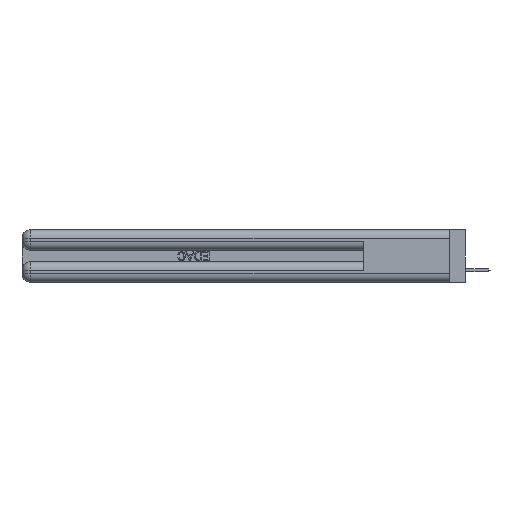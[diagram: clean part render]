
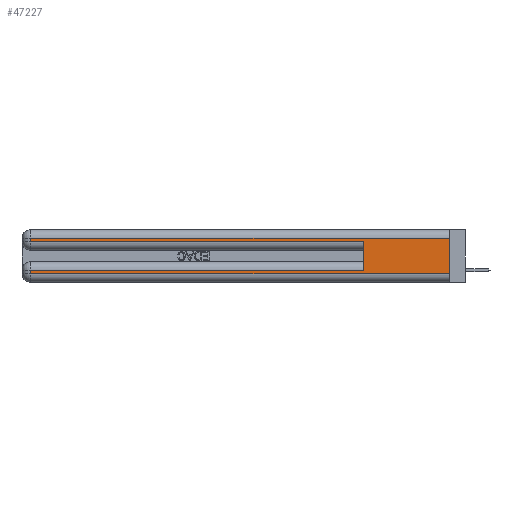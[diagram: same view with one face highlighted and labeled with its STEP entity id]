
A CAD part, left-side view. The second image highlights one B-rep face of the part: STEP entity #47227.
In plain terms, the highlighted planar face has unit normal (-1, 0, 0).
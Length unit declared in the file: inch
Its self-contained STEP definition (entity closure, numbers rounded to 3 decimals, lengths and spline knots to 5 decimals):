
#106 = CARTESIAN_POINT ( 'NONE',  ( 0., 0., 0.06 ) ) ;
#609 = VERTEX_POINT ( 'NONE', #6682 ) ;
#1346 = VERTEX_POINT ( 'NONE', #24670 ) ;
#2684 = EDGE_CURVE ( 'NONE', #16767, #4853, #29193, .T. ) ;
#2813 = CARTESIAN_POINT ( 'NONE',  ( 0., 0.6, 0.145 ) ) ;
#2814 = VERTEX_POINT ( 'NONE', #14439 ) ;
#3412 = CARTESIAN_POINT ( 'NONE',  ( 0., 0., 0.37 ) ) ;
#3419 = LINE ( 'NONE', #8866, #38883 ) ;
#4186 = CARTESIAN_POINT ( 'NONE',  ( 0., 2.94, 0.285 ) ) ;
#4853 = VERTEX_POINT ( 'NONE', #106 ) ;
#6113 = VECTOR ( 'NONE', #26702, 39.37008 ) ;
#6169 = ORIENTED_EDGE ( 'NONE', *, *, #49397, .T. ) ;
#6682 = CARTESIAN_POINT ( 'NONE',  ( 0., 0.6, 0.085 ) ) ;
#6764 = LINE ( 'NONE', #37122, #6113 ) ;
#7092 = LINE ( 'NONE', #46091, #16907 ) ;
#8866 = CARTESIAN_POINT ( 'NONE',  ( 0., 0., 0.085 ) ) ;
#12117 = VECTOR ( 'NONE', #26667, 39.37008 ) ;
#13129 = DIRECTION ( 'NONE',  ( 0., 1., 0. ) ) ;
#13929 = VECTOR ( 'NONE', #24621, 39.37008 ) ;
#14087 = CARTESIAN_POINT ( 'NONE',  ( 0., 0., 0.06 ) ) ;
#14439 = CARTESIAN_POINT ( 'NONE',  ( 0., 2.94, 0.31 ) ) ;
#15201 = PLANE ( 'NONE',  #41243 ) ;
#15898 = ORIENTED_EDGE ( 'NONE', *, *, #50608, .F. ) ;
#16653 = DIRECTION ( 'NONE',  ( 0., -1., 0. ) ) ;
#16767 = VERTEX_POINT ( 'NONE', #30334 ) ;
#16834 = CARTESIAN_POINT ( 'NONE',  ( 0., 0., 0.285 ) ) ;
#16907 = VECTOR ( 'NONE', #42018, 39.37008 ) ;
#16994 = ORIENTED_EDGE ( 'NONE', *, *, #35598, .T. ) ;
#17873 = ORIENTED_EDGE ( 'NONE', *, *, #2684, .T. ) ;
#17903 = FACE_OUTER_BOUND ( 'NONE', #39708, .T. ) ;
#18446 = EDGE_CURVE ( 'NONE', #609, #36268, #50624, .T. ) ;
#21858 = VECTOR ( 'NONE', #44849, 39.37008 ) ;
#22542 = LINE ( 'NONE', #24109, #12117 ) ;
#23091 = DIRECTION ( 'NONE',  ( 1., 0., 0. ) ) ;
#23515 = ORIENTED_EDGE ( 'NONE', *, *, #49285, .T. ) ;
#24109 = CARTESIAN_POINT ( 'NONE',  ( 0., 2.94, 0.37 ) ) ;
#24433 = CARTESIAN_POINT ( 'NONE',  ( 0., 0., 0.31 ) ) ;
#24621 = DIRECTION ( 'NONE',  ( 0., 0., -1. ) ) ;
#24670 = CARTESIAN_POINT ( 'NONE',  ( 0., 2.94, 0.085 ) ) ;
#26667 = DIRECTION ( 'NONE',  ( 0., 0., -1. ) ) ;
#26702 = DIRECTION ( 'NONE',  ( 0., 1., 0. ) ) ;
#27183 = EDGE_CURVE ( 'NONE', #609, #1346, #3419, .T. ) ;
#27396 = LINE ( 'NONE', #44066, #13929 ) ;
#27749 = VERTEX_POINT ( 'NONE', #4186 ) ;
#28210 = VECTOR ( 'NONE', #16653, 39.37008 ) ;
#29193 = LINE ( 'NONE', #14087, #21858 ) ;
#30334 = CARTESIAN_POINT ( 'NONE',  ( 0., 2.94, 0.06 ) ) ;
#30642 = VERTEX_POINT ( 'NONE', #24433 ) ;
#30935 = CARTESIAN_POINT ( 'NONE',  ( 0., 0.6, 0.285 ) ) ;
#35349 = EDGE_CURVE ( 'NONE', #27749, #36268, #38564, .T. ) ;
#35598 = EDGE_CURVE ( 'NONE', #30642, #2814, #6764, .T. ) ;
#36268 = VERTEX_POINT ( 'NONE', #30935 ) ;
#37122 = CARTESIAN_POINT ( 'NONE',  ( 0., 0., 0.31 ) ) ;
#37834 = DIRECTION ( 'NONE',  ( 0., 0., 1. ) ) ;
#38564 = LINE ( 'NONE', #16834, #28210 ) ;
#38789 = DIRECTION ( 'NONE',  ( 0., 0., -1. ) ) ;
#38883 = VECTOR ( 'NONE', #13129, 39.37008 ) ;
#39708 = EDGE_LOOP ( 'NONE', ( #15898, #16994, #6169, #42233, #46919, #42031, #23515, #17873 ) ) ;
#40266 = VECTOR ( 'NONE', #37834, 39.37008 ) ;
#41243 = AXIS2_PLACEMENT_3D ( 'NONE', #3412, #23091, #38789 ) ;
#42018 = DIRECTION ( 'NONE',  ( 0., 0., -1. ) ) ;
#42031 = ORIENTED_EDGE ( 'NONE', *, *, #27183, .T. ) ;
#42233 = ORIENTED_EDGE ( 'NONE', *, *, #35349, .T. ) ;
#44066 = CARTESIAN_POINT ( 'NONE',  ( 0., 2.94, 0.37 ) ) ;
#44849 = DIRECTION ( 'NONE',  ( 0., -1., 0. ) ) ;
#46091 = CARTESIAN_POINT ( 'NONE',  ( 0., 0., 0.37 ) ) ;
#46919 = ORIENTED_EDGE ( 'NONE', *, *, #18446, .F. ) ;
#47227 = ADVANCED_FACE ( 'NONE', ( #17903 ), #15201, .F. ) ;
#49285 = EDGE_CURVE ( 'NONE', #1346, #16767, #22542, .T. ) ;
#49397 = EDGE_CURVE ( 'NONE', #2814, #27749, #27396, .T. ) ;
#50608 = EDGE_CURVE ( 'NONE', #30642, #4853, #7092, .T. ) ;
#50624 = LINE ( 'NONE', #2813, #40266 ) ;
